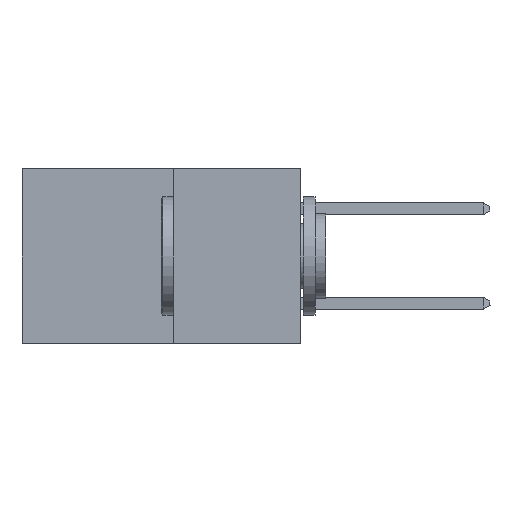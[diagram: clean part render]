
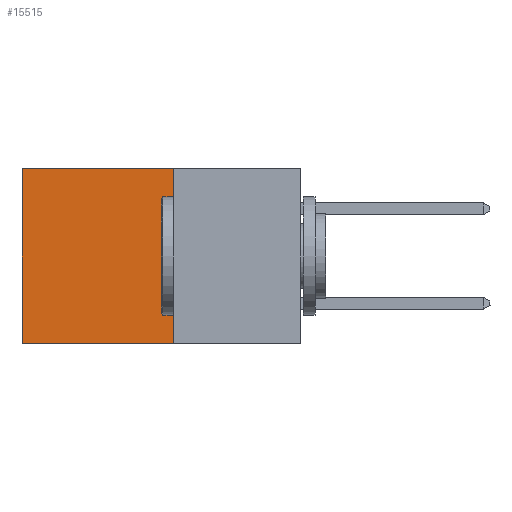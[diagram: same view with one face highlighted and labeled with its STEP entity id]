
A CAD part, left-side view. The second image highlights one B-rep face of the part: STEP entity #15515.
In plain terms, the highlighted planar face has unit normal (-1, 0, 0).
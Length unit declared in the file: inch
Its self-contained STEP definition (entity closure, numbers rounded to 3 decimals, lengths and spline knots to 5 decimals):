
#1514 = CARTESIAN_POINT ( 'NONE',  ( 0.277, 0.27, -0.37 ) ) ;
#1653 = DIRECTION ( 'NONE',  ( 0., 0., -1. ) ) ;
#2517 = VERTEX_POINT ( 'NONE', #14050 ) ;
#3221 = CARTESIAN_POINT ( 'NONE',  ( 0.277, 0.59, 0. ) ) ;
#4127 = VECTOR ( 'NONE', #24706, 39.37008 ) ;
#4263 = FACE_OUTER_BOUND ( 'NONE', #20412, .T. ) ;
#4966 = LINE ( 'NONE', #7384, #28878 ) ;
#5088 = VECTOR ( 'NONE', #19612, 39.37008 ) ;
#5370 = AXIS2_PLACEMENT_3D ( 'NONE', #26382, #15209, #1653 ) ;
#5693 = CARTESIAN_POINT ( 'NONE',  ( 0.277, 0.27, -0.37 ) ) ;
#5797 = LINE ( 'NONE', #1514, #5088 ) ;
#6923 = EDGE_CURVE ( 'NONE', #2517, #24121, #4966, .T. ) ;
#7384 = CARTESIAN_POINT ( 'NONE',  ( 0.277, 0.27, 0. ) ) ;
#8362 = CARTESIAN_POINT ( 'NONE',  ( 0.277, 0.59, -0.37 ) ) ;
#8654 = VERTEX_POINT ( 'NONE', #24094 ) ;
#11942 = DIRECTION ( 'NONE',  ( 0., 1., 0. ) ) ;
#12018 = EDGE_CURVE ( 'NONE', #2517, #8654, #21667, .T. ) ;
#12179 = VERTEX_POINT ( 'NONE', #8362 ) ;
#12940 = PLANE ( 'NONE',  #5370 ) ;
#14050 = CARTESIAN_POINT ( 'NONE',  ( 0.277, 0.27, 0. ) ) ;
#15209 = DIRECTION ( 'NONE',  ( 1., 0., 0. ) ) ;
#15515 = ADVANCED_FACE ( 'NONE', ( #4263 ), #12940, .F. ) ;
#15964 = ORIENTED_EDGE ( 'NONE', *, *, #17779, .T. ) ;
#16172 = LINE ( 'NONE', #22468, #4127 ) ;
#16392 = ORIENTED_EDGE ( 'NONE', *, *, #12018, .F. ) ;
#17779 = EDGE_CURVE ( 'NONE', #24121, #12179, #16172, .T. ) ;
#19612 = DIRECTION ( 'NONE',  ( 0., 1., 0. ) ) ;
#20412 = EDGE_LOOP ( 'NONE', ( #15964, #26808, #16392, #26635 ) ) ;
#21667 = LINE ( 'NONE', #5693, #27585 ) ;
#22468 = CARTESIAN_POINT ( 'NONE',  ( 0.277, 0.59, -0.37 ) ) ;
#23728 = DIRECTION ( 'NONE',  ( 0., 0., -1. ) ) ;
#24094 = CARTESIAN_POINT ( 'NONE',  ( 0.277, 0.27, -0.37 ) ) ;
#24121 = VERTEX_POINT ( 'NONE', #3221 ) ;
#24706 = DIRECTION ( 'NONE',  ( 0., 0., -1. ) ) ;
#26382 = CARTESIAN_POINT ( 'NONE',  ( 0.277, 0.27, -0.37 ) ) ;
#26635 = ORIENTED_EDGE ( 'NONE', *, *, #6923, .T. ) ;
#26808 = ORIENTED_EDGE ( 'NONE', *, *, #27903, .F. ) ;
#27585 = VECTOR ( 'NONE', #23728, 39.37008 ) ;
#27903 = EDGE_CURVE ( 'NONE', #8654, #12179, #5797, .T. ) ;
#28878 = VECTOR ( 'NONE', #11942, 39.37008 ) ;
